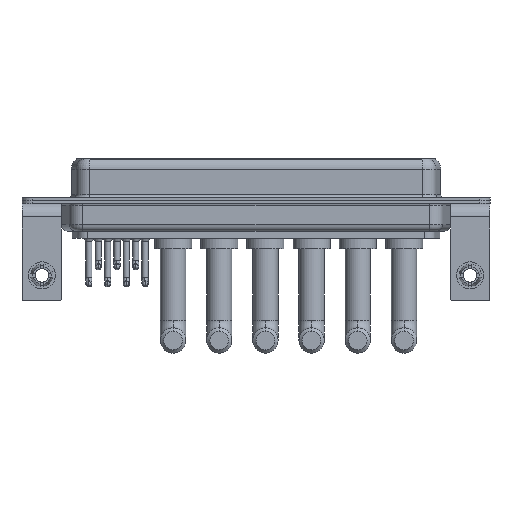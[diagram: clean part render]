
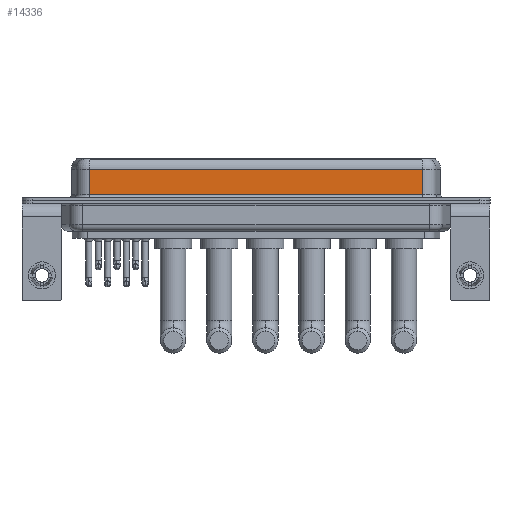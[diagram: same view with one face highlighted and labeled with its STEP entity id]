
A CAD part, front view. The second image highlights one B-rep face of the part: STEP entity #14336.
In plain terms, the highlighted planar face has unit normal (0, -1, 0).
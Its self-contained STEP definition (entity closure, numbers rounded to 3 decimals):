
#861 = CARTESIAN_POINT ( 'NONE',  ( 56.462, -3.95, 4.65 ) ) ;
#964 = LINE ( 'NONE', #861, #7130 ) ;
#1800 = CARTESIAN_POINT ( 'NONE',  ( 56.462, -3.95, 4.65 ) ) ;
#2143 = LINE ( 'NONE', #8574, #6604 ) ;
#2974 = EDGE_CURVE ( 'NONE', #4956, #19169, #964, .T. ) ;
#3546 = ORIENTED_EDGE ( 'NONE', *, *, #15973, .T. ) ;
#3636 = CARTESIAN_POINT ( 'NONE',  ( 7.038, -3.95, 0.9 ) ) ;
#4258 = DIRECTION ( 'NONE',  ( -1., 0., 0. ) ) ;
#4956 = VERTEX_POINT ( 'NONE', #1800 ) ;
#5646 = DIRECTION ( 'NONE',  ( 0., 0., 1. ) ) ;
#5747 = CARTESIAN_POINT ( 'NONE',  ( 56.462, -3.95, 6.4 ) ) ;
#5857 = LINE ( 'NONE', #12471, #9504 ) ;
#6466 = AXIS2_PLACEMENT_3D ( 'NONE', #5747, #15225, #5646 ) ;
#6604 = VECTOR ( 'NONE', #12609, 1000. ) ;
#6787 = CARTESIAN_POINT ( 'NONE',  ( 56.462, -3.95, 0.9 ) ) ;
#6816 = EDGE_CURVE ( 'NONE', #11830, #14708, #16083, .T. ) ;
#7130 = VECTOR ( 'NONE', #4258, 1000. ) ;
#7316 = EDGE_CURVE ( 'NONE', #4956, #14708, #2143, .T. ) ;
#8574 = CARTESIAN_POINT ( 'NONE',  ( 56.462, -3.95, 6.4 ) ) ;
#9232 = FACE_OUTER_BOUND ( 'NONE', #13897, .T. ) ;
#9315 = CARTESIAN_POINT ( 'NONE',  ( 7.038, -3.95, 4.65 ) ) ;
#9504 = VECTOR ( 'NONE', #17675, 1000. ) ;
#9691 = DIRECTION ( 'NONE',  ( 1., 0., 0. ) ) ;
#10591 = PLANE ( 'NONE',  #6466 ) ;
#11830 = VERTEX_POINT ( 'NONE', #3636 ) ;
#12471 = CARTESIAN_POINT ( 'NONE',  ( 7.038, -3.95, 6.4 ) ) ;
#12609 = DIRECTION ( 'NONE',  ( 0., 0., -1. ) ) ;
#13897 = EDGE_LOOP ( 'NONE', ( #18075, #14238, #3546, #18504 ) ) ;
#14238 = ORIENTED_EDGE ( 'NONE', *, *, #2974, .T. ) ;
#14336 = ADVANCED_FACE ( 'NONE', ( #9232 ), #10591, .F. ) ;
#14708 = VERTEX_POINT ( 'NONE', #6787 ) ;
#15225 = DIRECTION ( 'NONE',  ( 0., 1., 0. ) ) ;
#15973 = EDGE_CURVE ( 'NONE', #19169, #11830, #5857, .T. ) ;
#16083 = LINE ( 'NONE', #16187, #18645 ) ;
#16187 = CARTESIAN_POINT ( 'NONE',  ( 56.462, -3.95, 0.9 ) ) ;
#17675 = DIRECTION ( 'NONE',  ( 0., 0., -1. ) ) ;
#18075 = ORIENTED_EDGE ( 'NONE', *, *, #7316, .F. ) ;
#18504 = ORIENTED_EDGE ( 'NONE', *, *, #6816, .T. ) ;
#18645 = VECTOR ( 'NONE', #9691, 1000. ) ;
#19169 = VERTEX_POINT ( 'NONE', #9315 ) ;
